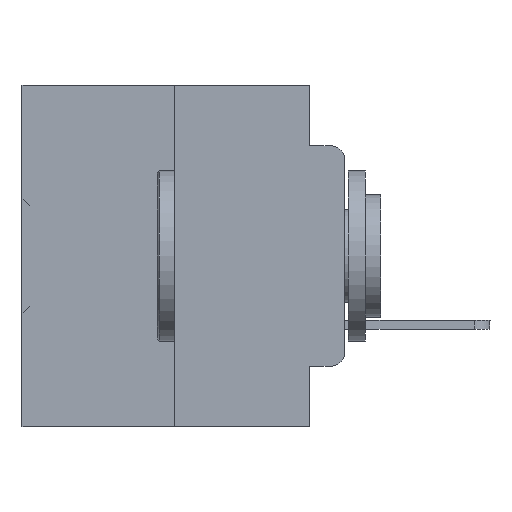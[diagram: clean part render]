
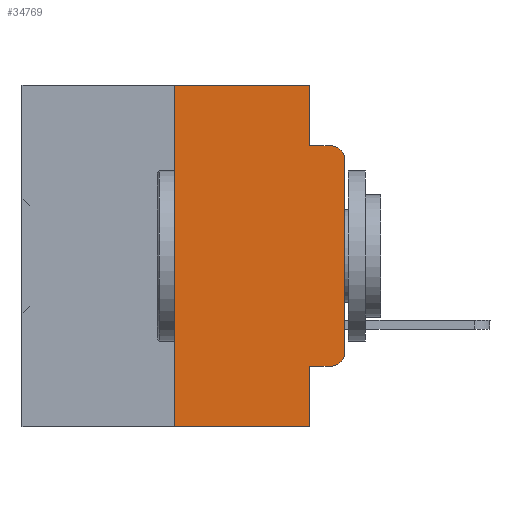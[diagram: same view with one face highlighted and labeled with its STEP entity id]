
A CAD part, left-side view. The second image highlights one B-rep face of the part: STEP entity #34769.
In plain terms, the highlighted planar face has unit normal (-1, 0, 0).
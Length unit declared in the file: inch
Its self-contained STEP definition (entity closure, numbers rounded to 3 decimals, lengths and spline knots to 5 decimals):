
#1630 = DIRECTION ( 'NONE',  ( 0., 0., 1. ) ) ;
#2180 = EDGE_CURVE ( 'NONE', #37938, #4933, #33991, .T. ) ;
#2602 = EDGE_CURVE ( 'NONE', #10115, #18097, #38100, .T. ) ;
#2872 = CARTESIAN_POINT ( 'NONE',  ( 0., 0.25, 0. ) ) ;
#3067 = EDGE_CURVE ( 'NONE', #27598, #25610, #16002, .T. ) ;
#3338 = VERTEX_POINT ( 'NONE', #21877 ) ;
#3550 = VECTOR ( 'NONE', #35825, 39.37008 ) ;
#3688 = DIRECTION ( 'NONE',  ( 0., -1., 0. ) ) ;
#3822 = CARTESIAN_POINT ( 'NONE',  ( 0., 0.051, -0.4115 ) ) ;
#3896 = ORIENTED_EDGE ( 'NONE', *, *, #2602, .F. ) ;
#4694 = VERTEX_POINT ( 'NONE', #15536 ) ;
#4725 = EDGE_CURVE ( 'NONE', #3338, #28414, #8425, .T. ) ;
#4933 = VERTEX_POINT ( 'NONE', #15794 ) ;
#5402 = EDGE_CURVE ( 'NONE', #10115, #37938, #38141, .T. ) ;
#5426 = LINE ( 'NONE', #23742, #3550 ) ;
#5960 = ORIENTED_EDGE ( 'NONE', *, *, #12207, .F. ) ;
#6468 = CARTESIAN_POINT ( 'NONE',  ( 0., 0.02, -0.1085 ) ) ;
#8083 = EDGE_CURVE ( 'NONE', #4694, #28414, #5426, .T. ) ;
#8425 = CIRCLE ( 'NONE', #30082, 0.02 ) ;
#9253 = DIRECTION ( 'NONE',  ( 0., 0., 1. ) ) ;
#9272 = EDGE_CURVE ( 'NONE', #25610, #31756, #13562, .T. ) ;
#10115 = VERTEX_POINT ( 'NONE', #10495 ) ;
#10495 = CARTESIAN_POINT ( 'NONE',  ( 0., 0.051, -0.4115 ) ) ;
#11374 = CARTESIAN_POINT ( 'NONE',  ( 0., 0.051, 0. ) ) ;
#11402 = ORIENTED_EDGE ( 'NONE', *, *, #8083, .F. ) ;
#12207 = EDGE_CURVE ( 'NONE', #31756, #4694, #25388, .T. ) ;
#12309 = VECTOR ( 'NONE', #21587, 39.37008 ) ;
#12704 = DIRECTION ( 'NONE',  ( 0., 0., -1. ) ) ;
#13071 = LINE ( 'NONE', #19289, #21880 ) ;
#13124 = CARTESIAN_POINT ( 'NONE',  ( 0., 0.051, -0.5 ) ) ;
#13562 = LINE ( 'NONE', #17889, #26016 ) ;
#13718 = ORIENTED_EDGE ( 'NONE', *, *, #19212, .T. ) ;
#14395 = CARTESIAN_POINT ( 'NONE',  ( 0., 0.02, -0.0885 ) ) ;
#14550 = CARTESIAN_POINT ( 'NONE',  ( 0., 0.02, -0.3915 ) ) ;
#15536 = CARTESIAN_POINT ( 'NONE',  ( 0., 0.051, -0.0885 ) ) ;
#15794 = CARTESIAN_POINT ( 'NONE',  ( 0., 0., -0.3915 ) ) ;
#16002 = LINE ( 'NONE', #2872, #17371 ) ;
#16751 = ORIENTED_EDGE ( 'NONE', *, *, #5402, .T. ) ;
#17258 = DIRECTION ( 'NONE',  ( 0., 0., -1. ) ) ;
#17371 = VECTOR ( 'NONE', #9253, 39.37008 ) ;
#17398 = VECTOR ( 'NONE', #32183, 39.37008 ) ;
#17889 = CARTESIAN_POINT ( 'NONE',  ( 0., 0.473, 0. ) ) ;
#18097 = VERTEX_POINT ( 'NONE', #13124 ) ;
#19212 = EDGE_CURVE ( 'NONE', #4933, #3338, #13071, .T. ) ;
#19289 = CARTESIAN_POINT ( 'NONE',  ( 0., 0., 0. ) ) ;
#19820 = ORIENTED_EDGE ( 'NONE', *, *, #9272, .F. ) ;
#20912 = DIRECTION ( 'NONE',  ( 0., -1., 0. ) ) ;
#21587 = DIRECTION ( 'NONE',  ( 0., -1., 0. ) ) ;
#21877 = CARTESIAN_POINT ( 'NONE',  ( 0., 0., -0.1085 ) ) ;
#21880 = VECTOR ( 'NONE', #1630, 39.37008 ) ;
#22043 = EDGE_LOOP ( 'NONE', ( #13718, #26661, #11402, #5960, #19820, #25416, #25523, #3896, #16751, #23481 ) ) ;
#23481 = ORIENTED_EDGE ( 'NONE', *, *, #2180, .T. ) ;
#23742 = CARTESIAN_POINT ( 'NONE',  ( 0., 0.051, -0.0885 ) ) ;
#25388 = LINE ( 'NONE', #11374, #17398 ) ;
#25416 = ORIENTED_EDGE ( 'NONE', *, *, #3067, .F. ) ;
#25523 = ORIENTED_EDGE ( 'NONE', *, *, #33106, .T. ) ;
#25610 = VERTEX_POINT ( 'NONE', #37523 ) ;
#26016 = VECTOR ( 'NONE', #20912, 39.37008 ) ;
#26661 = ORIENTED_EDGE ( 'NONE', *, *, #4725, .T. ) ;
#27563 = CARTESIAN_POINT ( 'NONE',  ( 0., 0.473, 0. ) ) ;
#27598 = VERTEX_POINT ( 'NONE', #37240 ) ;
#27682 = CARTESIAN_POINT ( 'NONE',  ( 0., 0.02, -0.4115 ) ) ;
#28414 = VERTEX_POINT ( 'NONE', #14395 ) ;
#29120 = AXIS2_PLACEMENT_3D ( 'NONE', #27563, #36745, #36877 ) ;
#29199 = DIRECTION ( 'NONE',  ( 0., 0., -1. ) ) ;
#30082 = AXIS2_PLACEMENT_3D ( 'NONE', #6468, #30278, #12704 ) ;
#30273 = VECTOR ( 'NONE', #3688, 39.37008 ) ;
#30278 = DIRECTION ( 'NONE',  ( -1., 0., 0. ) ) ;
#31756 = VERTEX_POINT ( 'NONE', #35728 ) ;
#32183 = DIRECTION ( 'NONE',  ( 0., 0., -1. ) ) ;
#32242 = FACE_OUTER_BOUND ( 'NONE', #22043, .T. ) ;
#32498 = AXIS2_PLACEMENT_3D ( 'NONE', #14550, #35512, #17258 ) ;
#33106 = EDGE_CURVE ( 'NONE', #27598, #18097, #33737, .T. ) ;
#33737 = LINE ( 'NONE', #36273, #12309 ) ;
#33991 = CIRCLE ( 'NONE', #32498, 0.02 ) ;
#34769 = ADVANCED_FACE ( 'NONE', ( #32242 ), #36357, .F. ) ;
#35512 = DIRECTION ( 'NONE',  ( -1., 0., 0. ) ) ;
#35728 = CARTESIAN_POINT ( 'NONE',  ( 0., 0.051, 0. ) ) ;
#35825 = DIRECTION ( 'NONE',  ( 0., -1., 0. ) ) ;
#36273 = CARTESIAN_POINT ( 'NONE',  ( 0., 0.473, -0.5 ) ) ;
#36357 = PLANE ( 'NONE',  #29120 ) ;
#36745 = DIRECTION ( 'NONE',  ( 1., 0., 0. ) ) ;
#36877 = DIRECTION ( 'NONE',  ( 0., 0., -1. ) ) ;
#37200 = VECTOR ( 'NONE', #29199, 39.37008 ) ;
#37240 = CARTESIAN_POINT ( 'NONE',  ( 0., 0.25, -0.5 ) ) ;
#37523 = CARTESIAN_POINT ( 'NONE',  ( 0., 0.25, 0. ) ) ;
#37938 = VERTEX_POINT ( 'NONE', #27682 ) ;
#37988 = CARTESIAN_POINT ( 'NONE',  ( 0., 0.051, 0. ) ) ;
#38100 = LINE ( 'NONE', #37988, #37200 ) ;
#38141 = LINE ( 'NONE', #3822, #30273 ) ;
